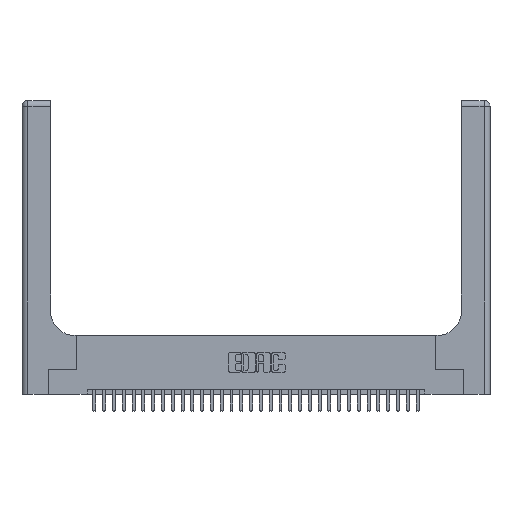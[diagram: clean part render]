
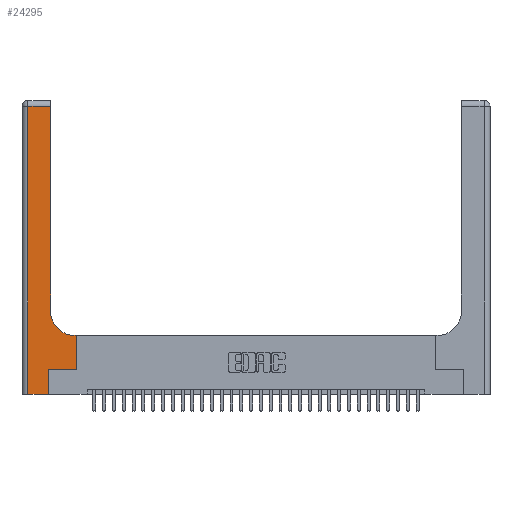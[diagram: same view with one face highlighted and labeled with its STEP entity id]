
A CAD part, top view. The second image highlights one B-rep face of the part: STEP entity #24295.
In plain terms, the highlighted planar face has unit normal (0, 0, 1).
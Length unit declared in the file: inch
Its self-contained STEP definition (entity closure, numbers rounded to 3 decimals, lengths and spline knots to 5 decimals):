
#114 = ORIENTED_EDGE ( 'NONE', *, *, #21335, .T. ) ;
#151 = CARTESIAN_POINT ( 'NONE',  ( 0.5585, 0.25, 0.37 ) ) ;
#898 = CARTESIAN_POINT ( 'NONE',  ( 0.06, 2.94, 0.37 ) ) ;
#1055 = CARTESIAN_POINT ( 'NONE',  ( 0.5585, 0.6, 0.37 ) ) ;
#1517 = VERTEX_POINT ( 'NONE', #18190 ) ;
#1594 = CARTESIAN_POINT ( 'NONE',  ( 0.269, 0.25, 0.37 ) ) ;
#2373 = VECTOR ( 'NONE', #5660, 39.37008 ) ;
#3580 = EDGE_CURVE ( 'NONE', #1517, #14410, #9368, .T. ) ;
#3607 = VECTOR ( 'NONE', #24277, 39.37008 ) ;
#3921 = CARTESIAN_POINT ( 'NONE',  ( 0.269, 0., 0.37 ) ) ;
#4761 = DIRECTION ( 'NONE',  ( 1., 0., 0. ) ) ;
#4921 = VERTEX_POINT ( 'NONE', #13440 ) ;
#5660 = DIRECTION ( 'NONE',  ( 0., 1., 0. ) ) ;
#5661 = ORIENTED_EDGE ( 'NONE', *, *, #16254, .T. ) ;
#6800 = LINE ( 'NONE', #19409, #3607 ) ;
#7891 = DIRECTION ( 'NONE',  ( 0., 0., -1. ) ) ;
#7964 = CARTESIAN_POINT ( 'NONE',  ( 0., 0., 0.37 ) ) ;
#8450 = ORIENTED_EDGE ( 'NONE', *, *, #30416, .T. ) ;
#9368 = CIRCLE ( 'NONE', #29934, 0.25 ) ;
#9617 = CARTESIAN_POINT ( 'NONE',  ( 0.06, 3., 0.37 ) ) ;
#9924 = LINE ( 'NONE', #23368, #2373 ) ;
#10050 = EDGE_LOOP ( 'NONE', ( #20495, #15430, #29242, #8450, #31348, #5661, #114, #16710, #17185 ) ) ;
#10463 = DIRECTION ( 'NONE',  ( -1., 0., 0. ) ) ;
#11698 = VERTEX_POINT ( 'NONE', #898 ) ;
#11884 = DIRECTION ( 'NONE',  ( 0., 1., 0. ) ) ;
#11988 = CARTESIAN_POINT ( 'NONE',  ( 0.5415, 0.85, 0.37 ) ) ;
#12225 = EDGE_CURVE ( 'NONE', #11698, #18773, #25241, .T. ) ;
#13440 = CARTESIAN_POINT ( 'NONE',  ( 0.2915, 2.94, 0.37 ) ) ;
#14029 = VECTOR ( 'NONE', #30614, 39.37008 ) ;
#14231 = VERTEX_POINT ( 'NONE', #1055 ) ;
#14410 = VERTEX_POINT ( 'NONE', #18227 ) ;
#14452 = DIRECTION ( 'NONE',  ( 0., -1., 0. ) ) ;
#15011 = DIRECTION ( 'NONE',  ( 1., 0., 0. ) ) ;
#15430 = ORIENTED_EDGE ( 'NONE', *, *, #19259, .T. ) ;
#15545 = AXIS2_PLACEMENT_3D ( 'NONE', #23149, #7891, #10463 ) ;
#16254 = EDGE_CURVE ( 'NONE', #18120, #32371, #22151, .T. ) ;
#16710 = ORIENTED_EDGE ( 'NONE', *, *, #25573, .T. ) ;
#17185 = ORIENTED_EDGE ( 'NONE', *, *, #3580, .T. ) ;
#18074 = PLANE ( 'NONE',  #15545 ) ;
#18120 = VERTEX_POINT ( 'NONE', #1594 ) ;
#18190 = CARTESIAN_POINT ( 'NONE',  ( 0.5415, 0.6, 0.37 ) ) ;
#18227 = CARTESIAN_POINT ( 'NONE',  ( 0.2915, 0.85, 0.37 ) ) ;
#18429 = CARTESIAN_POINT ( 'NONE',  ( 0.06, 0., 0.37 ) ) ;
#18773 = VERTEX_POINT ( 'NONE', #18429 ) ;
#18913 = EDGE_CURVE ( 'NONE', #14410, #4921, #25613, .T. ) ;
#19259 = EDGE_CURVE ( 'NONE', #4921, #11698, #6800, .T. ) ;
#19409 = CARTESIAN_POINT ( 'NONE',  ( 0., 2.94, 0.37 ) ) ;
#19426 = CARTESIAN_POINT ( 'NONE',  ( 0.269, 0.25, 0.37 ) ) ;
#19785 = VERTEX_POINT ( 'NONE', #3921 ) ;
#19825 = CARTESIAN_POINT ( 'NONE',  ( 0.2915, 3., 0.37 ) ) ;
#20164 = VECTOR ( 'NONE', #22280, 39.37008 ) ;
#20495 = ORIENTED_EDGE ( 'NONE', *, *, #18913, .T. ) ;
#21335 = EDGE_CURVE ( 'NONE', #32371, #14231, #9924, .T. ) ;
#21449 = VECTOR ( 'NONE', #21910, 39.37008 ) ;
#21910 = DIRECTION ( 'NONE',  ( 0., 1., 0. ) ) ;
#22151 = LINE ( 'NONE', #19426, #20164 ) ;
#22280 = DIRECTION ( 'NONE',  ( 1., 0., 0. ) ) ;
#23013 = LINE ( 'NONE', #29444, #21449 ) ;
#23149 = CARTESIAN_POINT ( 'NONE',  ( 0., 3., 0.37 ) ) ;
#23368 = CARTESIAN_POINT ( 'NONE',  ( 0.5585, 0.25, 0.37 ) ) ;
#23572 = VECTOR ( 'NONE', #14452, 39.37008 ) ;
#23959 = LINE ( 'NONE', #33072, #14029 ) ;
#24277 = DIRECTION ( 'NONE',  ( -1., 0., 0. ) ) ;
#24295 = ADVANCED_FACE ( 'NONE', ( #32109 ), #18074, .F. ) ;
#25241 = LINE ( 'NONE', #9617, #23572 ) ;
#25573 = EDGE_CURVE ( 'NONE', #14231, #1517, #23959, .T. ) ;
#25613 = LINE ( 'NONE', #19825, #29215 ) ;
#25645 = LINE ( 'NONE', #7964, #28059 ) ;
#26723 = EDGE_CURVE ( 'NONE', #19785, #18120, #23013, .T. ) ;
#28059 = VECTOR ( 'NONE', #4761, 39.37008 ) ;
#29215 = VECTOR ( 'NONE', #11884, 39.37008 ) ;
#29242 = ORIENTED_EDGE ( 'NONE', *, *, #12225, .T. ) ;
#29444 = CARTESIAN_POINT ( 'NONE',  ( 0.269, 0., 0.37 ) ) ;
#29934 = AXIS2_PLACEMENT_3D ( 'NONE', #11988, #32667, #15011 ) ;
#30416 = EDGE_CURVE ( 'NONE', #18773, #19785, #25645, .T. ) ;
#30614 = DIRECTION ( 'NONE',  ( -1., 0., 0. ) ) ;
#31348 = ORIENTED_EDGE ( 'NONE', *, *, #26723, .T. ) ;
#32109 = FACE_OUTER_BOUND ( 'NONE', #10050, .T. ) ;
#32371 = VERTEX_POINT ( 'NONE', #151 ) ;
#32667 = DIRECTION ( 'NONE',  ( 0., 0., -1. ) ) ;
#33072 = CARTESIAN_POINT ( 'NONE',  ( 0.2915, 0.6, 0.37 ) ) ;
